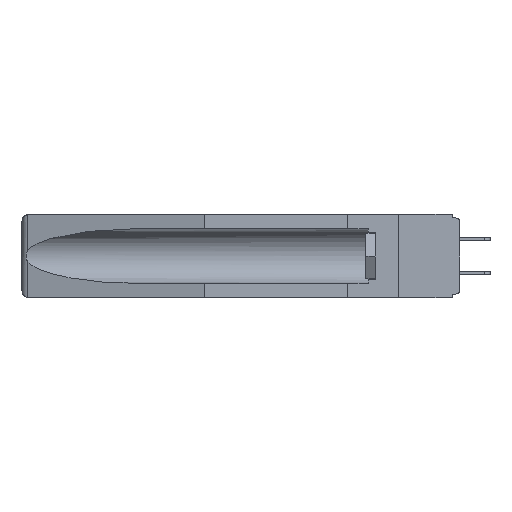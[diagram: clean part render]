
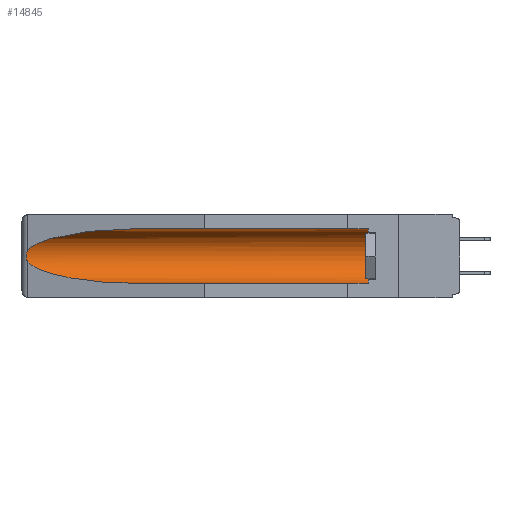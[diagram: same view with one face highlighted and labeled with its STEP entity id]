
A CAD part, left-side view. The second image highlights one B-rep face of the part: STEP entity #14845.
In plain terms, the highlighted cylindrical face has radius 2.857 mm (diameter 5.715 mm), a partial arc.
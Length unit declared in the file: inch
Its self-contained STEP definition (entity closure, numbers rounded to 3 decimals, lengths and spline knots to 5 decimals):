
#149 = CARTESIAN_POINT ( 'NONE',  ( 0.26537, 1.52718, -0.19328 ) ) ;
#661 = CARTESIAN_POINT ( 'NONE',  ( 0.26537, 1.52718, -0.14972 ) ) ;
#781 = ORIENTED_EDGE ( 'NONE', *, *, #8616, .T. ) ;
#934 = CARTESIAN_POINT ( 'NONE',  ( 0.155, 1.07973, -0.059 ) ) ;
#1188 = CARTESIAN_POINT ( 'NONE',  ( 0.26654, 1.53092, -0.15636 ) ) ;
#1396 = CARTESIAN_POINT ( 'NONE',  ( 0.2673, 1.53269, -0.17917 ) ) ;
#2418 = CARTESIAN_POINT ( 'NONE',  ( 0.155, 0.126, -0.059 ) ) ;
#2449 = DIRECTION ( 'NONE',  ( 0., 0., 1. ) ) ;
#2732 = CARTESIAN_POINT ( 'NONE',  ( 0.26537, 1.52718, -0.14972 ) ) ;
#2771 = CARTESIAN_POINT ( 'NONE',  ( 0.21114, 1.30732, -0.059 ) ) ;
#2949 = CARTESIAN_POINT ( 'NONE',  ( 0.26537, 1.52718, -0.19328 ) ) ;
#2983 = CARTESIAN_POINT ( 'NONE',  ( 0.25451, 1.48313, -0.24835 ) ) ;
#3428 =( BOUNDED_CURVE ( )  B_SPLINE_CURVE ( 3, ( #17653, #2983, #6303, #9399 ),
 .UNSPECIFIED., .F., .F. ) 
 B_SPLINE_CURVE_WITH_KNOTS ( ( 4, 4 ),
 ( 0.1948, 1.5708 ),
 .UNSPECIFIED. ) 
 CURVE ( )  GEOMETRIC_REPRESENTATION_ITEM ( )  RATIONAL_B_SPLINE_CURVE ( ( 1., 0.848, 0.848, 1. ) ) 
 REPRESENTATION_ITEM ( '' )  );
#3667 = EDGE_LOOP ( 'NONE', ( #13393, #11492, #9277, #13693, #781, #17946 ) ) ;
#3992 = CARTESIAN_POINT ( 'NONE',  ( 0.155, -0.30754, -0.1715 ) ) ;
#4104 = CIRCLE ( 'NONE', #16508, 0.1125 ) ;
#4351 = CARTESIAN_POINT ( 'NONE',  ( 0.26655, 1.53094, -0.18657 ) ) ;
#5244 = CARTESIAN_POINT ( 'NONE',  ( 0.155, -0.30754, -0.284 ) ) ;
#5497 = DIRECTION ( 'NONE',  ( 0., 0., 1. ) ) ;
#5702 = DIRECTION ( 'NONE',  ( 0., -1., 0. ) ) ;
#5958 = CARTESIAN_POINT ( 'NONE',  ( 0.26537, 1.52718, -0.14972 ) ) ;
#6064 = CARTESIAN_POINT ( 'NONE',  ( 0.26597, 1.52961, -0.15275 ) ) ;
#6303 = CARTESIAN_POINT ( 'NONE',  ( 0.21114, 1.30732, -0.284 ) ) ;
#6711 = LINE ( 'NONE', #5244, #15521 ) ;
#6713 = EDGE_CURVE ( 'NONE', #15834, #15647, #12770, .T. ) ;
#6916 = VERTEX_POINT ( 'NONE', #8545 ) ;
#7004 = DIRECTION ( 'NONE',  ( 0., 1., 0. ) ) ;
#7114 = DIRECTION ( 'NONE',  ( 0., 1., 0. ) ) ;
#7197 = B_SPLINE_CURVE_WITH_KNOTS ( 'NONE', 3,
 ( #2732, #6064, #1188, #11055, #15849, #17404, #1396, #4351, #12670, #2949 ),
 .UNSPECIFIED., .F., .F.,
 ( 4, 2, 2, 2, 4 ),
 ( 0., 0.00029, 0.00058, 0.00087, 0.00117 ),
 .UNSPECIFIED. ) ;
#7396 = DIRECTION ( 'NONE',  ( 0., 1., 0. ) ) ;
#8545 = CARTESIAN_POINT ( 'NONE',  ( 0.155, 0.126, -0.284 ) ) ;
#8616 = EDGE_CURVE ( 'NONE', #6916, #17909, #4104, .T. ) ;
#8889 = CARTESIAN_POINT ( 'NONE',  ( 0.155, 1.07973, -0.284 ) ) ;
#9277 = ORIENTED_EDGE ( 'NONE', *, *, #9791, .T. ) ;
#9334 = CARTESIAN_POINT ( 'NONE',  ( 0.155, 1.07973, -0.059 ) ) ;
#9399 = CARTESIAN_POINT ( 'NONE',  ( 0.155, 1.07973, -0.284 ) ) ;
#9557 = AXIS2_PLACEMENT_3D ( 'NONE', #3992, #7114, #2449 ) ;
#9791 = EDGE_CURVE ( 'NONE', #13031, #11372, #3428, .T. ) ;
#10440 = VECTOR ( 'NONE', #7396, 39.37008 ) ;
#10689 = FACE_OUTER_BOUND ( 'NONE', #3667, .T. ) ;
#11055 = CARTESIAN_POINT ( 'NONE',  ( 0.2673, 1.5327, -0.16383 ) ) ;
#11372 = VERTEX_POINT ( 'NONE', #8889 ) ;
#11492 = ORIENTED_EDGE ( 'NONE', *, *, #17409, .T. ) ;
#12401 = CARTESIAN_POINT ( 'NONE',  ( 0.155, -0.30754, -0.059 ) ) ;
#12670 = CARTESIAN_POINT ( 'NONE',  ( 0.26597, 1.5296, -0.19026 ) ) ;
#12770 =( BOUNDED_CURVE ( )  B_SPLINE_CURVE ( 3, ( #9334, #2771, #20631, #5958 ),
 .UNSPECIFIED., .F., .F. ) 
 B_SPLINE_CURVE_WITH_KNOTS ( ( 4, 4 ),
 ( 4.71239, 6.08839 ),
 .UNSPECIFIED. ) 
 CURVE ( )  GEOMETRIC_REPRESENTATION_ITEM ( )  RATIONAL_B_SPLINE_CURVE ( ( 1., 0.848, 0.848, 1. ) ) 
 REPRESENTATION_ITEM ( '' )  );
#13031 = VERTEX_POINT ( 'NONE', #149 ) ;
#13393 = ORIENTED_EDGE ( 'NONE', *, *, #6713, .T. ) ;
#13693 = ORIENTED_EDGE ( 'NONE', *, *, #15599, .F. ) ;
#14845 = ADVANCED_FACE ( 'NONE', ( #10689 ), #17770, .F. ) ;
#15521 = VECTOR ( 'NONE', #7004, 39.37008 ) ;
#15599 = EDGE_CURVE ( 'NONE', #6916, #11372, #6711, .T. ) ;
#15647 = VERTEX_POINT ( 'NONE', #661 ) ;
#15834 = VERTEX_POINT ( 'NONE', #934 ) ;
#15849 = CARTESIAN_POINT ( 'NONE',  ( 0.2675, 1.53308, -0.16763 ) ) ;
#16288 = EDGE_CURVE ( 'NONE', #17909, #15834, #19056, .T. ) ;
#16508 = AXIS2_PLACEMENT_3D ( 'NONE', #18678, #5702, #5497 ) ;
#17404 = CARTESIAN_POINT ( 'NONE',  ( 0.2675, 1.53308, -0.17534 ) ) ;
#17409 = EDGE_CURVE ( 'NONE', #15647, #13031, #7197, .T. ) ;
#17653 = CARTESIAN_POINT ( 'NONE',  ( 0.26537, 1.52718, -0.19328 ) ) ;
#17770 = CYLINDRICAL_SURFACE ( 'NONE', #9557, 0.1125 ) ;
#17909 = VERTEX_POINT ( 'NONE', #2418 ) ;
#17946 = ORIENTED_EDGE ( 'NONE', *, *, #16288, .T. ) ;
#18678 = CARTESIAN_POINT ( 'NONE',  ( 0.155, 0.126, -0.1715 ) ) ;
#19056 = LINE ( 'NONE', #12401, #10440 ) ;
#20631 = CARTESIAN_POINT ( 'NONE',  ( 0.25451, 1.48313, -0.09465 ) ) ;
